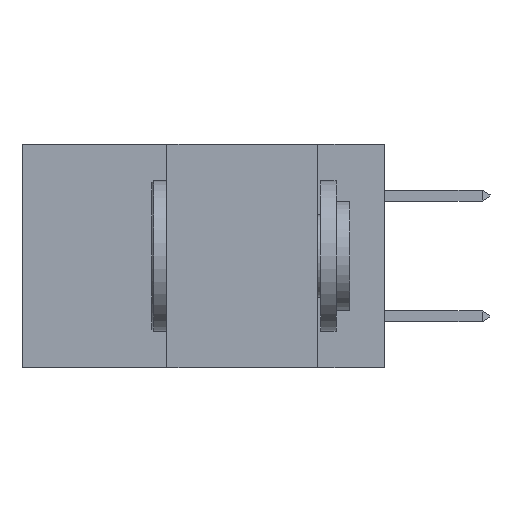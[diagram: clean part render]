
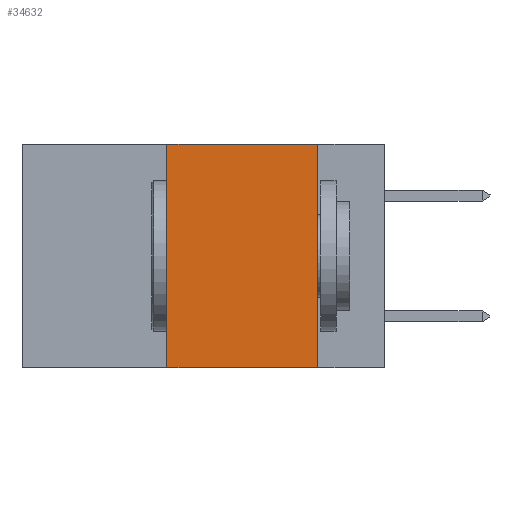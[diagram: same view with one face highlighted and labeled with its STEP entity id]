
A CAD part, left-side view. The second image highlights one B-rep face of the part: STEP entity #34632.
In plain terms, the highlighted planar face has unit normal (-1, 0, 0).
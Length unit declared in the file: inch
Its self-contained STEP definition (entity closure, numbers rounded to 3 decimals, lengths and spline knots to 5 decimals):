
#4201 = VERTEX_POINT ( 'NONE', #26119 ) ;
#4332 = EDGE_CURVE ( 'NONE', #25385, #13449, #20080, .T. ) ;
#4956 = CARTESIAN_POINT ( 'NONE',  ( 0., 0.6, 0. ) ) ;
#4959 = DIRECTION ( 'NONE',  ( 0., 0., -1. ) ) ;
#5919 = VECTOR ( 'NONE', #28106, 39.37008 ) ;
#6757 = LINE ( 'NONE', #13216, #8534 ) ;
#6982 = LINE ( 'NONE', #4956, #12659 ) ;
#7344 = CARTESIAN_POINT ( 'NONE',  ( 0., 0.6, 0. ) ) ;
#8534 = VECTOR ( 'NONE', #4959, 39.37008 ) ;
#9134 = ORIENTED_EDGE ( 'NONE', *, *, #30894, .T. ) ;
#10393 = CARTESIAN_POINT ( 'NONE',  ( 0., 0.11, 0. ) ) ;
#11434 = ORIENTED_EDGE ( 'NONE', *, *, #4332, .F. ) ;
#11737 = CARTESIAN_POINT ( 'NONE',  ( 0., 0.36, -0.37 ) ) ;
#11880 = VECTOR ( 'NONE', #15792, 39.37008 ) ;
#12659 = VECTOR ( 'NONE', #16022, 39.37008 ) ;
#12939 = DIRECTION ( 'NONE',  ( 1., 0., 0. ) ) ;
#12976 = CARTESIAN_POINT ( 'NONE',  ( 0., 0.36, 0. ) ) ;
#13216 = CARTESIAN_POINT ( 'NONE',  ( 0., 0.11, 0. ) ) ;
#13449 = VERTEX_POINT ( 'NONE', #22458 ) ;
#15792 = DIRECTION ( 'NONE',  ( 0., 0., 1. ) ) ;
#16022 = DIRECTION ( 'NONE',  ( 0., -1., 0. ) ) ;
#20080 = LINE ( 'NONE', #12976, #11880 ) ;
#22214 = ORIENTED_EDGE ( 'NONE', *, *, #23150, .F. ) ;
#22458 = CARTESIAN_POINT ( 'NONE',  ( 0., 0.36, 0. ) ) ;
#23150 = EDGE_CURVE ( 'NONE', #25922, #4201, #6757, .T. ) ;
#23933 = AXIS2_PLACEMENT_3D ( 'NONE', #7344, #12939, #33319 ) ;
#25353 = CARTESIAN_POINT ( 'NONE',  ( 0., 0.6, -0.37 ) ) ;
#25385 = VERTEX_POINT ( 'NONE', #11737 ) ;
#25922 = VERTEX_POINT ( 'NONE', #10393 ) ;
#26119 = CARTESIAN_POINT ( 'NONE',  ( 0., 0.11, -0.37 ) ) ;
#27113 = EDGE_CURVE ( 'NONE', #13449, #25922, #6982, .T. ) ;
#27950 = LINE ( 'NONE', #25353, #5919 ) ;
#28106 = DIRECTION ( 'NONE',  ( 0., -1., 0. ) ) ;
#28243 = EDGE_LOOP ( 'NONE', ( #22214, #35292, #11434, #9134 ) ) ;
#29380 = PLANE ( 'NONE',  #23933 ) ;
#29848 = FACE_OUTER_BOUND ( 'NONE', #28243, .T. ) ;
#30894 = EDGE_CURVE ( 'NONE', #25385, #4201, #27950, .T. ) ;
#33319 = DIRECTION ( 'NONE',  ( 0., 0., -1. ) ) ;
#34632 = ADVANCED_FACE ( 'NONE', ( #29848 ), #29380, .F. ) ;
#35292 = ORIENTED_EDGE ( 'NONE', *, *, #27113, .F. ) ;
